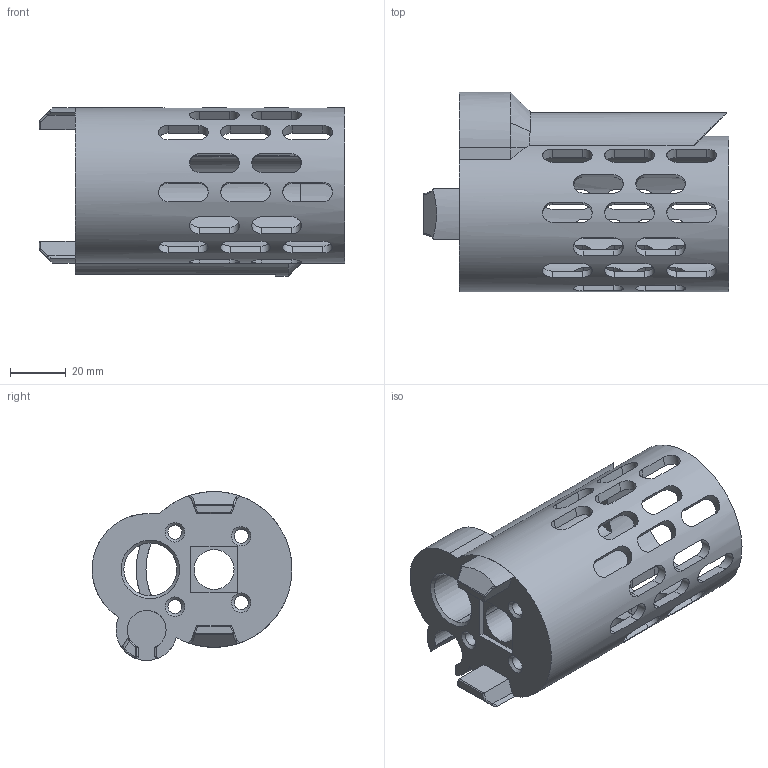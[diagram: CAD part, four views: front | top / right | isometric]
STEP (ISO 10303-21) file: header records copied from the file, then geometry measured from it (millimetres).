
FILE_DESCRIPTION(/* description */ (''),/* implementation_level */ '2;1');
FILE_NAME(/* name */ 'MOD9_GOAT_TEC_barrel_retainer v8.step',/* time_stamp */ '2020-07-19T19:16:09-05:00',/* author */ (''),/* organization */ (''),/* preprocessor_version */ 'ST-DEVELOPER v18.1',/* originating_system */ 'Autodesk Translation Framework v9.3.0.1241',/* authorisation */ '');
FILE_SCHEMA (('AUTOMOTIVE_DESIGN { 1 0 10303 214 3 1 1 }'));
Length unit declared in the file: millimetre
Products named in the file (1): MOD9_GOAT_TEC_barrel_retainer
Bounding box: 110.02 x 71.88 x 60.72 mm (x, y, z)
Volume: 105306.4 mm3; surface area: 43288.7 mm2
Topology: 1 solids, 1 shells, 231 faces, 657 edges, 425 vertices
Faces by surface type: cylinder 107, plane 97, cone 9, bspline 8, sphere 6, torus 4
Full cylindrical faces by diameter (mm): 5 x4, 49 x1, 56 x1
Entity records: 9658 total; most frequent: CARTESIAN_POINT 3748, ORIENTED_EDGE 1312, DIRECTION 1053, EDGE_CURVE 656, VERTEX_POINT 425, LINE 371, VECTOR 371, AXIS2_PLACEMENT_3D 341
